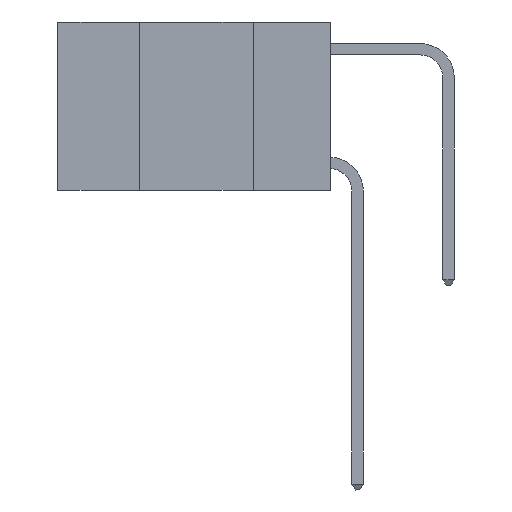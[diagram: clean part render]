
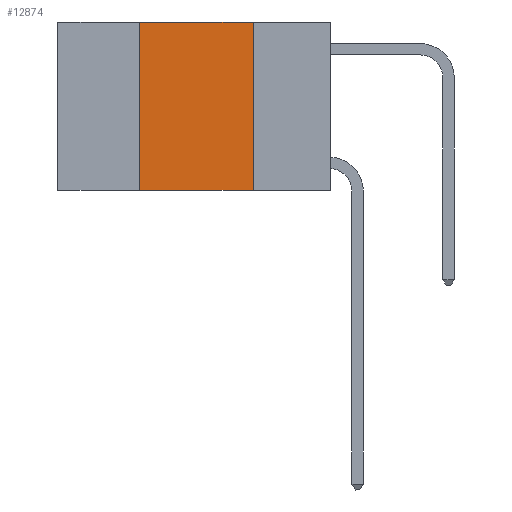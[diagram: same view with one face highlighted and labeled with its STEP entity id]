
A CAD part, left-side view. The second image highlights one B-rep face of the part: STEP entity #12874.
In plain terms, the highlighted planar face has unit normal (-1, 0, 0).
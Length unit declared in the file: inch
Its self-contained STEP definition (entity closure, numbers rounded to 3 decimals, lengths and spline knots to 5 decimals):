
#595 = AXIS2_PLACEMENT_3D ( 'NONE', #4692, #9539, #10468 ) ;
#712 = FACE_OUTER_BOUND ( 'NONE', #11910, .T. ) ;
#717 = VERTEX_POINT ( 'NONE', #7270 ) ;
#786 = DIRECTION ( 'NONE',  ( 0., -1., 0. ) ) ;
#1264 = EDGE_CURVE ( 'NONE', #1702, #11288, #9599, .T. ) ;
#1702 = VERTEX_POINT ( 'NONE', #2470 ) ;
#2286 = VECTOR ( 'NONE', #786, 39.37008 ) ;
#2343 = EDGE_CURVE ( 'NONE', #717, #4983, #8901, .T. ) ;
#2470 = CARTESIAN_POINT ( 'NONE',  ( 0., 0.42, 0. ) ) ;
#3062 = LINE ( 'NONE', #4011, #4439 ) ;
#3869 = CARTESIAN_POINT ( 'NONE',  ( 0., 0.17, 0. ) ) ;
#4011 = CARTESIAN_POINT ( 'NONE',  ( 0., 0.17, 0. ) ) ;
#4141 = ORIENTED_EDGE ( 'NONE', *, *, #9613, .F. ) ;
#4439 = VECTOR ( 'NONE', #4879, 39.37008 ) ;
#4496 = CARTESIAN_POINT ( 'NONE',  ( 0., 0.42, 0. ) ) ;
#4692 = CARTESIAN_POINT ( 'NONE',  ( 0., 0.6, 0. ) ) ;
#4879 = DIRECTION ( 'NONE',  ( 0., 0., -1. ) ) ;
#4983 = VERTEX_POINT ( 'NONE', #11840 ) ;
#5605 = CARTESIAN_POINT ( 'NONE',  ( 0., 0.6, 0. ) ) ;
#6549 = EDGE_CURVE ( 'NONE', #717, #1702, #10427, .T. ) ;
#7134 = ORIENTED_EDGE ( 'NONE', *, *, #1264, .F. ) ;
#7270 = CARTESIAN_POINT ( 'NONE',  ( 0., 0.42, -0.37 ) ) ;
#7462 = DIRECTION ( 'NONE',  ( 0., 0., 1. ) ) ;
#8609 = VECTOR ( 'NONE', #7462, 39.37008 ) ;
#8719 = ORIENTED_EDGE ( 'NONE', *, *, #2343, .T. ) ;
#8901 = LINE ( 'NONE', #11831, #2286 ) ;
#9539 = DIRECTION ( 'NONE',  ( 1., 0., 0. ) ) ;
#9599 = LINE ( 'NONE', #5605, #10380 ) ;
#9613 = EDGE_CURVE ( 'NONE', #11288, #4983, #3062, .T. ) ;
#10380 = VECTOR ( 'NONE', #12344, 39.37008 ) ;
#10427 = LINE ( 'NONE', #4496, #8609 ) ;
#10468 = DIRECTION ( 'NONE',  ( 0., 0., -1. ) ) ;
#11288 = VERTEX_POINT ( 'NONE', #3869 ) ;
#11386 = PLANE ( 'NONE',  #595 ) ;
#11831 = CARTESIAN_POINT ( 'NONE',  ( 0., 0.6, -0.37 ) ) ;
#11840 = CARTESIAN_POINT ( 'NONE',  ( 0., 0.17, -0.37 ) ) ;
#11910 = EDGE_LOOP ( 'NONE', ( #4141, #7134, #12729, #8719 ) ) ;
#12344 = DIRECTION ( 'NONE',  ( 0., -1., 0. ) ) ;
#12729 = ORIENTED_EDGE ( 'NONE', *, *, #6549, .F. ) ;
#12874 = ADVANCED_FACE ( 'NONE', ( #712 ), #11386, .F. ) ;
